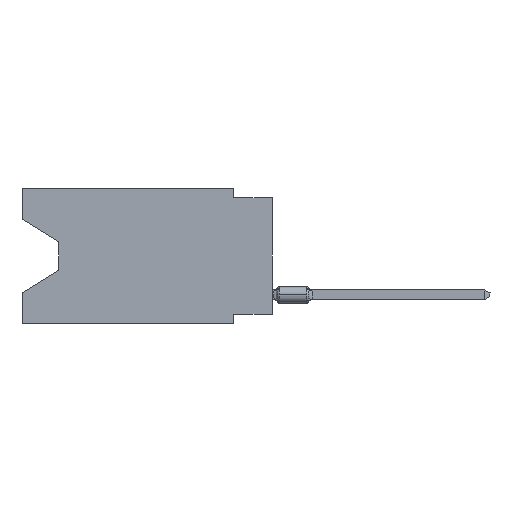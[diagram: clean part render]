
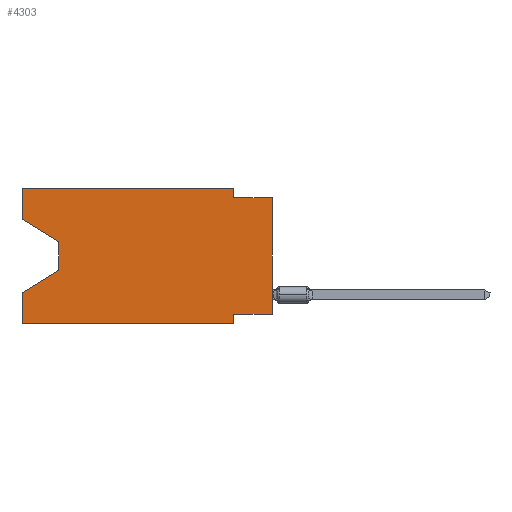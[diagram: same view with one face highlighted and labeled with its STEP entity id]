
A CAD part, left-side view. The second image highlights one B-rep face of the part: STEP entity #4303.
In plain terms, the highlighted planar face has unit normal (-1, 0, 0).
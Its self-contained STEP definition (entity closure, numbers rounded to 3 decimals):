
#23 = DIRECTION ( 'NONE',  ( 0., 0., 1. ) ) ;
#1802 = VERTEX_POINT ( 'NONE', #14816 ) ;
#2065 = CARTESIAN_POINT ( 'NONE',  ( 0., 2.54, -0.635 ) ) ;
#2183 = DIRECTION ( 'NONE',  ( 0., 0., -1. ) ) ;
#2832 = VERTEX_POINT ( 'NONE', #51390 ) ;
#3103 = CARTESIAN_POINT ( 'NONE',  ( 0., 13.97, -3.505 ) ) ;
#4140 = CARTESIAN_POINT ( 'NONE',  ( 0., 16.383, 0. ) ) ;
#4303 = ADVANCED_FACE ( 'NONE', ( #26976 ), #75874, .F. ) ;
#5237 = ORIENTED_EDGE ( 'NONE', *, *, #86821, .T. ) ;
#6191 = CARTESIAN_POINT ( 'NONE',  ( 0., 0., -8.255 ) ) ;
#6745 = CARTESIAN_POINT ( 'NONE',  ( 0., 13.97, -5.385 ) ) ;
#6978 = LINE ( 'NONE', #35395, #91253 ) ;
#7178 = AXIS2_PLACEMENT_3D ( 'NONE', #4140, #68889, #55404 ) ;
#7269 = DIRECTION ( 'NONE',  ( 0., 0., 1. ) ) ;
#7364 = LINE ( 'NONE', #35790, #20347 ) ;
#7796 = CARTESIAN_POINT ( 'NONE',  ( 0., 0., -0.635 ) ) ;
#7890 = EDGE_CURVE ( 'NONE', #31627, #1802, #53409, .T. ) ;
#8362 = EDGE_LOOP ( 'NONE', ( #62592, #5237, #53105, #15644, #64383, #48625, #77879, #78517, #88765, #86859, #63537, #32613 ) ) ;
#11621 = VECTOR ( 'NONE', #47688, 1000. ) ;
#14816 = CARTESIAN_POINT ( 'NONE',  ( 0., 16.383, -6.852 ) ) ;
#15644 = ORIENTED_EDGE ( 'NONE', *, *, #7890, .F. ) ;
#16645 = CARTESIAN_POINT ( 'NONE',  ( 0., 16.383, -8.89 ) ) ;
#18821 = LINE ( 'NONE', #47244, #74414 ) ;
#19342 = DIRECTION ( 'NONE',  ( 0., -1., 0. ) ) ;
#20347 = VECTOR ( 'NONE', #86977, 1000. ) ;
#24164 = VERTEX_POINT ( 'NONE', #86930 ) ;
#24735 = DIRECTION ( 'NONE',  ( 0., 0., -1. ) ) ;
#25315 = VERTEX_POINT ( 'NONE', #79057 ) ;
#26976 = FACE_OUTER_BOUND ( 'NONE', #8362, .T. ) ;
#27791 = LINE ( 'NONE', #34773, #51345 ) ;
#31627 = VERTEX_POINT ( 'NONE', #16645 ) ;
#31977 = DIRECTION ( 'NONE',  ( 0., 0., 1. ) ) ;
#32370 = VERTEX_POINT ( 'NONE', #7796 ) ;
#32613 = ORIENTED_EDGE ( 'NONE', *, *, #56275, .F. ) ;
#32875 = EDGE_CURVE ( 'NONE', #2832, #35327, #82038, .T. ) ;
#34572 = VERTEX_POINT ( 'NONE', #6191 ) ;
#34773 = CARTESIAN_POINT ( 'NONE',  ( 0., 16.383, 0. ) ) ;
#35327 = VERTEX_POINT ( 'NONE', #68273 ) ;
#35395 = CARTESIAN_POINT ( 'NONE',  ( 0., 0., 0. ) ) ;
#35790 = CARTESIAN_POINT ( 'NONE',  ( 0., 16.383, -8.89 ) ) ;
#38095 = DIRECTION ( 'NONE',  ( 0., -1., 0. ) ) ;
#38281 = CARTESIAN_POINT ( 'NONE',  ( 0., 2.54, -8.89 ) ) ;
#38750 = DIRECTION ( 'NONE',  ( 0., 0., -1. ) ) ;
#39380 = LINE ( 'NONE', #6745, #88888 ) ;
#39829 = VECTOR ( 'NONE', #19342, 1000. ) ;
#39837 = LINE ( 'NONE', #53377, #39829 ) ;
#40098 = CARTESIAN_POINT ( 'NONE',  ( 0., 2.54, 0. ) ) ;
#41152 = VECTOR ( 'NONE', #38750, 1000. ) ;
#47244 = CARTESIAN_POINT ( 'NONE',  ( 0., 16.383, -2.038 ) ) ;
#47688 = DIRECTION ( 'NONE',  ( 0., 1., 0. ) ) ;
#48625 = ORIENTED_EDGE ( 'NONE', *, *, #32875, .F. ) ;
#49119 = DIRECTION ( 'NONE',  ( 0., -0.855, -0.519 ) ) ;
#51345 = VECTOR ( 'NONE', #7269, 1000. ) ;
#51390 = CARTESIAN_POINT ( 'NONE',  ( 0., 2.54, -8.255 ) ) ;
#53105 = ORIENTED_EDGE ( 'NONE', *, *, #66184, .T. ) ;
#53377 = CARTESIAN_POINT ( 'NONE',  ( 0., 0., -0.635 ) ) ;
#53409 = LINE ( 'NONE', #82255, #62515 ) ;
#53636 = LINE ( 'NONE', #40098, #74119 ) ;
#55161 = CARTESIAN_POINT ( 'NONE',  ( 0., 0., -8.255 ) ) ;
#55404 = DIRECTION ( 'NONE',  ( 0., 0., -1. ) ) ;
#56275 = EDGE_CURVE ( 'NONE', #25315, #75411, #27791, .T. ) ;
#57498 = VERTEX_POINT ( 'NONE', #58129 ) ;
#58129 = CARTESIAN_POINT ( 'NONE',  ( 0., 13.97, -3.505 ) ) ;
#59810 = EDGE_CURVE ( 'NONE', #31627, #35327, #7364, .T. ) ;
#61191 = LINE ( 'NONE', #55161, #11621 ) ;
#62165 = VECTOR ( 'NONE', #38095, 1000. ) ;
#62403 = CARTESIAN_POINT ( 'NONE',  ( 0., 16.383, 0. ) ) ;
#62515 = VECTOR ( 'NONE', #31977, 1000. ) ;
#62592 = ORIENTED_EDGE ( 'NONE', *, *, #70399, .T. ) ;
#63537 = ORIENTED_EDGE ( 'NONE', *, *, #74428, .F. ) ;
#64383 = ORIENTED_EDGE ( 'NONE', *, *, #59810, .T. ) ;
#66147 = EDGE_CURVE ( 'NONE', #67562, #32370, #39837, .T. ) ;
#66184 = EDGE_CURVE ( 'NONE', #70555, #1802, #39380, .T. ) ;
#67374 = LINE ( 'NONE', #3103, #80160 ) ;
#67562 = VERTEX_POINT ( 'NONE', #2065 ) ;
#68273 = CARTESIAN_POINT ( 'NONE',  ( 0., 2.54, -8.89 ) ) ;
#68889 = DIRECTION ( 'NONE',  ( 1., 0., 0. ) ) ;
#68956 = EDGE_CURVE ( 'NONE', #34572, #2832, #61191, .T. ) ;
#70399 = EDGE_CURVE ( 'NONE', #25315, #57498, #18821, .T. ) ;
#70555 = VERTEX_POINT ( 'NONE', #78423 ) ;
#71480 = DIRECTION ( 'NONE',  ( 0., 0.855, -0.519 ) ) ;
#74119 = VECTOR ( 'NONE', #24735, 1000. ) ;
#74414 = VECTOR ( 'NONE', #49119, 1000. ) ;
#74428 = EDGE_CURVE ( 'NONE', #75411, #24164, #82303, .T. ) ;
#75411 = VERTEX_POINT ( 'NONE', #62403 ) ;
#75874 = PLANE ( 'NONE',  #7178 ) ;
#77879 = ORIENTED_EDGE ( 'NONE', *, *, #68956, .F. ) ;
#78423 = CARTESIAN_POINT ( 'NONE',  ( 0., 13.97, -5.385 ) ) ;
#78517 = ORIENTED_EDGE ( 'NONE', *, *, #78905, .T. ) ;
#78905 = EDGE_CURVE ( 'NONE', #34572, #32370, #6978, .T. ) ;
#79057 = CARTESIAN_POINT ( 'NONE',  ( 0., 16.383, -2.038 ) ) ;
#80160 = VECTOR ( 'NONE', #2183, 1000. ) ;
#80476 = CARTESIAN_POINT ( 'NONE',  ( 0., 16.383, 0. ) ) ;
#82038 = LINE ( 'NONE', #38281, #41152 ) ;
#82255 = CARTESIAN_POINT ( 'NONE',  ( 0., 16.383, 0. ) ) ;
#82303 = LINE ( 'NONE', #80476, #62165 ) ;
#86554 = EDGE_CURVE ( 'NONE', #24164, #67562, #53636, .T. ) ;
#86821 = EDGE_CURVE ( 'NONE', #57498, #70555, #67374, .T. ) ;
#86859 = ORIENTED_EDGE ( 'NONE', *, *, #86554, .F. ) ;
#86930 = CARTESIAN_POINT ( 'NONE',  ( 0., 2.54, 0. ) ) ;
#86977 = DIRECTION ( 'NONE',  ( 0., -1., 0. ) ) ;
#88765 = ORIENTED_EDGE ( 'NONE', *, *, #66147, .F. ) ;
#88888 = VECTOR ( 'NONE', #71480, 1000. ) ;
#91253 = VECTOR ( 'NONE', #23, 1000. ) ;
